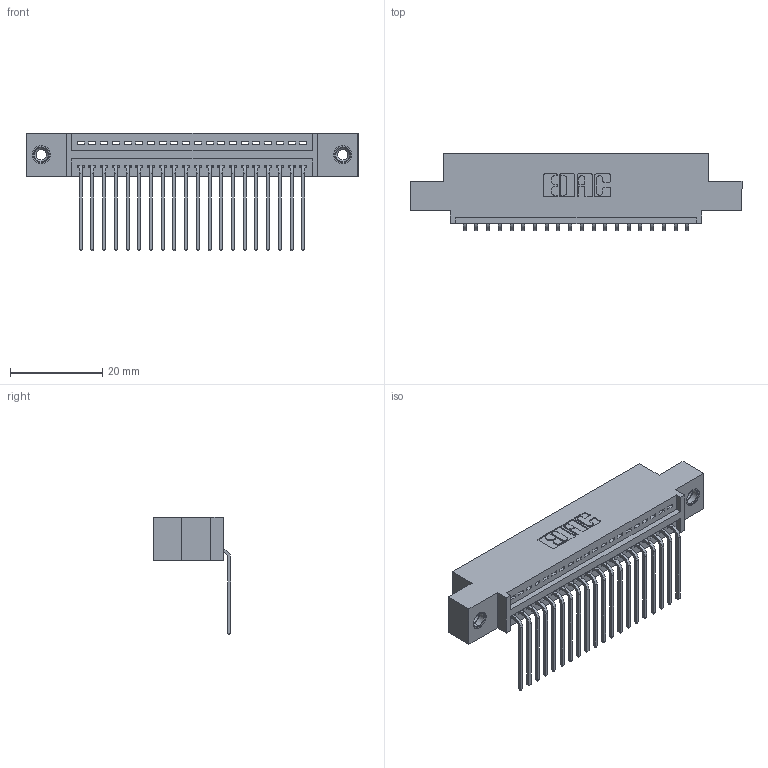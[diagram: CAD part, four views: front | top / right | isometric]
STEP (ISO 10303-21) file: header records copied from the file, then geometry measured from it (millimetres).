
FILE_DESCRIPTION (( 'STEP AP203' ), '1' );
FILE_NAME ('345-020-559-408.STEP', '2019-10-04T21:25:19', ( '' ), ( '' ), 'SwSTEP 2.0', 'SolidWorks 2016', '' );
FILE_SCHEMA (( 'CONFIG_CONTROL_DESIGN' ));
Length unit declared in the file: inch
Products named in the file (4): 345 Part_0.110 Offset - 0.156 Dia-TI; 345-250-001_345-250-003-102; 345-020-559-408; 345-292-001_558 559 Tail - 1
Assembly tree (23 placements, depth 2):
  345-020-559-408
    345 Part_0.110 Offset - 0.156 Dia-TI
    345-292-001_558 559 Tail - 1  x20
    345-250-001_345-250-003-102  x2
Bounding box: 72.01 x 16.75 x 25.53 mm (x, y, z)
Volume: 6646 mm3; surface area: 9025.6 mm2
Topology: 23 solids, 23 shells, 1390 faces, 4129 edges, 2718 vertices
Faces by surface type: plane 956, cylinder 418, cone 12, torus 4
Entity records: 19416 total; most frequent: CARTESIAN_POINT 3347, ORIENTED_EDGE 3294, DIRECTION 2981, EDGE_CURVE 1647, LINE 1415, VECTOR 1415, VERTEX_POINT 1092, AXIS2_PLACEMENT_3D 783
